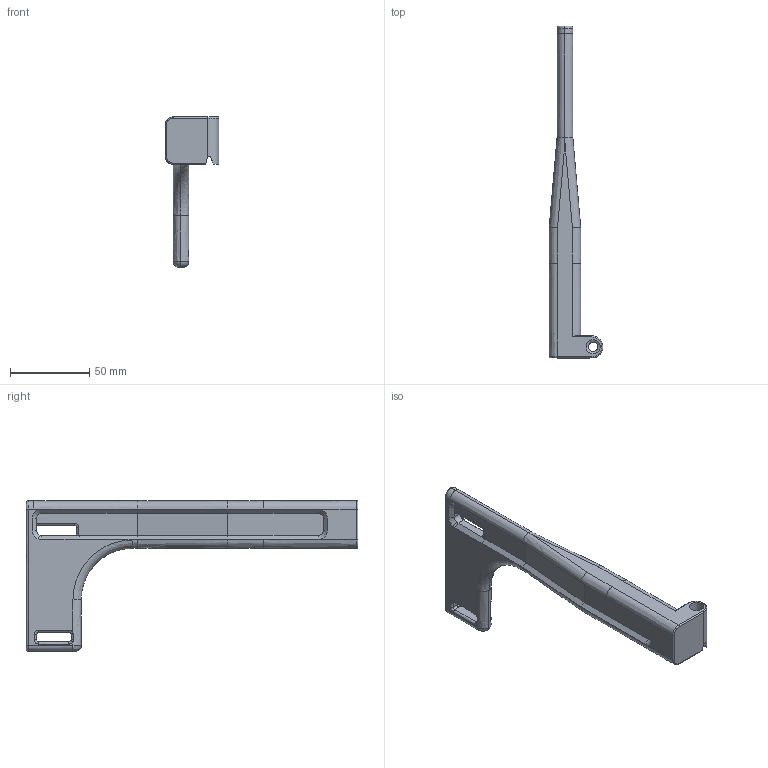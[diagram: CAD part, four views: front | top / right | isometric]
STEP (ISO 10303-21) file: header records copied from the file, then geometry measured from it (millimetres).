
FILE_DESCRIPTION(/* description */ (''),/* implementation_level */ '2;1');
FILE_NAME(/* name */ 'Brace V2.step',/* time_stamp */ '2021-02-07T17:44:13-07:00',/* author */ (''),/* organization */ (''),/* preprocessor_version */ 'ST-DEVELOPER v18.1',/* originating_system */ 'Autodesk Translation Framework v9.7.1.1290',/* authorisation */ '');
FILE_SCHEMA (('AUTOMOTIVE_DESIGN { 1 0 10303 214 3 1 1 }'));
Length unit declared in the file: inch
Products named in the file (1): Brace V2
Bounding box: 34 x 210 x 95 mm (x, y, z)
Volume: 102348.3 mm3; surface area: 26469.7 mm2
Topology: 1 solids, 1 shells, 161 faces, 413 edges, 249 vertices
Faces by surface type: bspline 66, plane 55, cylinder 24, cone 9, torus 7
Full cylindrical faces by diameter (mm): 6 x1, 9 x1
Entity records: 7184 total; most frequent: CARTESIAN_POINT 3758, ORIENTED_EDGE 826, DIRECTION 494, EDGE_CURVE 413, VERTEX_POINT 249, B_SPLINE_CURVE_WITH_KNOTS 184, AXIS2_PLACEMENT_3D 169, EDGE_LOOP 162
